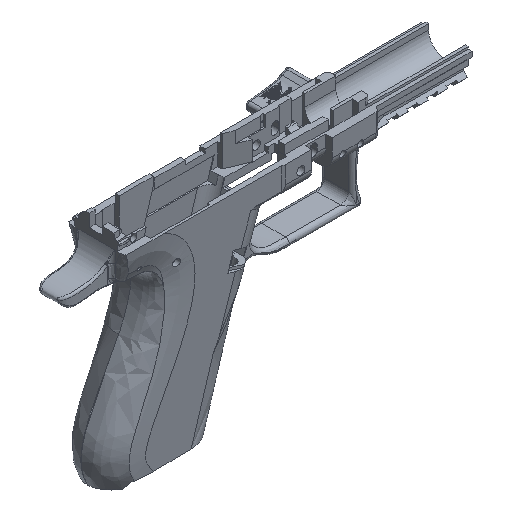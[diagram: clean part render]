
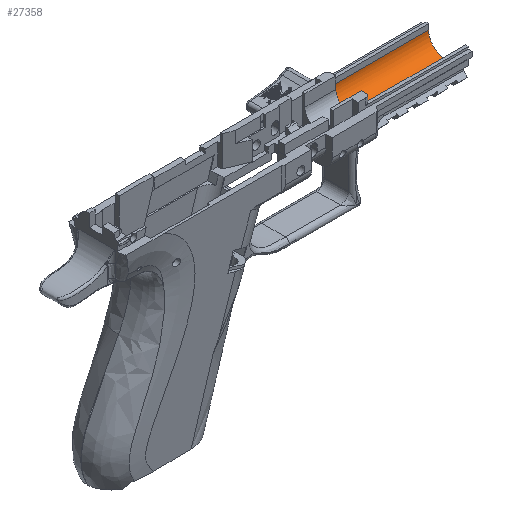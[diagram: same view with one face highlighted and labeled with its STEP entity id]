
A CAD part, isometric view. The second image highlights one B-rep face of the part: STEP entity #27358.
In plain terms, the highlighted cylindrical face has radius 8.75 mm (diameter 17.5 mm), a partial arc.
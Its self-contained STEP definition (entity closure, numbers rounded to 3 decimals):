
#133=CYLINDRICAL_SURFACE('',#28163,8.75);
#3768=LINE('',#60984,#5748);
#3770=LINE('',#60994,#5750);
#5748=VECTOR('',#31421,1000.);
#5750=VECTOR('',#31425,1000.);
#7587=FACE_OUTER_BOUND('',#9077,.T.);
#9077=EDGE_LOOP('',(#25024,#25025,#25026,#25027,#25028));
#9388=CIRCLE('',#28027,8.75);
#9416=CIRCLE('',#28164,8.75);
#10506=B_SPLINE_CURVE_WITH_KNOTS('',3,(#60987,#60988,#60989,#60990,#60991,
#60992),.UNSPECIFIED.,.F.,.F.,(4,2,4),(0.734,0.932,
1.014),.UNSPECIFIED.);
#13099=VERTEX_POINT('',#60287);
#13100=VERTEX_POINT('',#60288);
#13261=VERTEX_POINT('',#60981);
#13262=VERTEX_POINT('',#60983);
#13263=VERTEX_POINT('',#60993);
#17030=EDGE_CURVE('',#13099,#13100,#9388,.T.);
#17313=EDGE_CURVE('',#13262,#13261,#3768,.T.);
#17315=EDGE_CURVE('',#13261,#13099,#10506,.T.);
#17316=EDGE_CURVE('',#13263,#13100,#3770,.T.);
#17317=EDGE_CURVE('',#13262,#13263,#9416,.T.);
#25024=ORIENTED_EDGE('',*,*,#17313,.T.);
#25025=ORIENTED_EDGE('',*,*,#17315,.T.);
#25026=ORIENTED_EDGE('',*,*,#17030,.T.);
#25027=ORIENTED_EDGE('',*,*,#17316,.F.);
#25028=ORIENTED_EDGE('',*,*,#17317,.F.);
#27358=ADVANCED_FACE('',(#7587),#133,.F.);
#28027=AXIS2_PLACEMENT_3D('',#60289,#30916,#30917);
#28163=AXIS2_PLACEMENT_3D('',#60986,#31423,#31424);
#28164=AXIS2_PLACEMENT_3D('',#60995,#31426,#31427);
#30916=DIRECTION('center_axis',(-1.,0.,0.));
#30917=DIRECTION('ref_axis',(0.,-1.,0.));
#31421=DIRECTION('',(-1.,0.,0.));
#31423=DIRECTION('center_axis',(-1.,0.,0.));
#31424=DIRECTION('ref_axis',(0.,-1.,0.));
#31425=DIRECTION('',(-1.,0.,0.));
#31426=DIRECTION('center_axis',(-1.,0.,0.));
#31427=DIRECTION('ref_axis',(0.,-1.,0.));
#60287=CARTESIAN_POINT('',(128.4,33.743,102.843));
#60288=CARTESIAN_POINT('',(128.4,25.493,97.009));
#60289=CARTESIAN_POINT('Origin',(128.4,25.493,105.759));
#60981=CARTESIAN_POINT('',(128.336,34.243,105.759));
#60983=CARTESIAN_POINT('',(178.4,34.243,105.759));
#60984=CARTESIAN_POINT('',(178.4,34.243,105.759));
#60986=CARTESIAN_POINT('Origin',(178.4,25.493,105.759));
#60987=CARTESIAN_POINT('Ctrl Pts',(128.336,34.243,105.759));
#60988=CARTESIAN_POINT('Ctrl Pts',(128.336,34.243,105.099));
#60989=CARTESIAN_POINT('Ctrl Pts',(128.363,34.163,104.382));
#60990=CARTESIAN_POINT('Ctrl Pts',(128.393,33.924,103.402));
#60991=CARTESIAN_POINT('Ctrl Pts',(128.4,33.84,103.118));
#60992=CARTESIAN_POINT('Ctrl Pts',(128.4,33.743,102.843));
#60993=CARTESIAN_POINT('',(178.4,25.493,97.009));
#60994=CARTESIAN_POINT('',(178.4,25.493,97.009));
#60995=CARTESIAN_POINT('Origin',(178.4,25.493,105.759));
